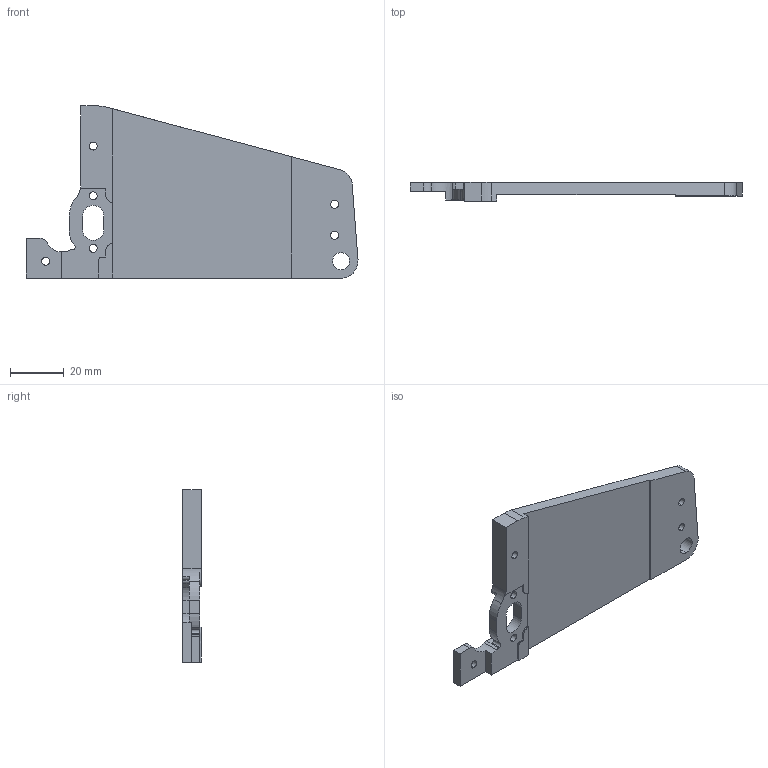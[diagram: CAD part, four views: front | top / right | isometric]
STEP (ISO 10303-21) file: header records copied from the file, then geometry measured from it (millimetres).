
FILE_DESCRIPTION (( 'STEP AP214' ), '1' );
FILE_NAME ('Thunderbolt_Mag_Well_Right.STEP', '2021-09-12T03:38:54', ( '' ), ( '' ), 'SwSTEP 2.0', 'SolidWorks 2020', '' );
FILE_SCHEMA (( 'AUTOMOTIVE_DESIGN' ));
Length unit declared in the file: millimetre
Products named in the file (1): Thunderbolt_Mag_Well_Right
Bounding box: 124.11 x 7.03 x 64.36 mm (x, y, z)
Volume: 23872.5 mm3; surface area: 15162.1 mm2
Topology: 1 solids, 1 shells, 298 faces, 828 edges, 552 vertices
Faces by surface type: plane 175, bspline 77, cylinder 46
Entity records: 12200 total; most frequent: CARTESIAN_POINT 4924, ORIENTED_EDGE 1656, DIRECTION 1214, EDGE_CURVE 828, LINE 578, VECTOR 578, VERTEX_POINT 552, EDGE_LOOP 334
